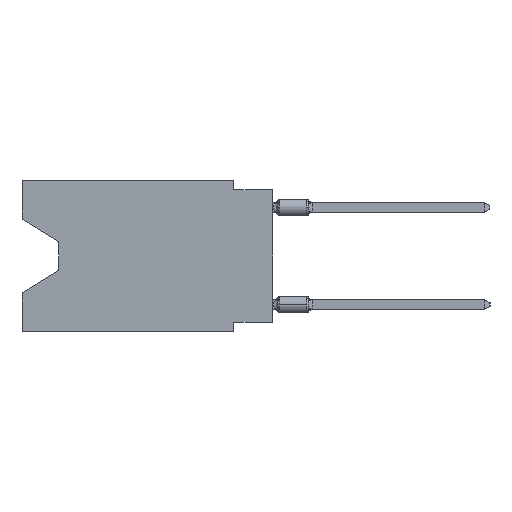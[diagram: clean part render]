
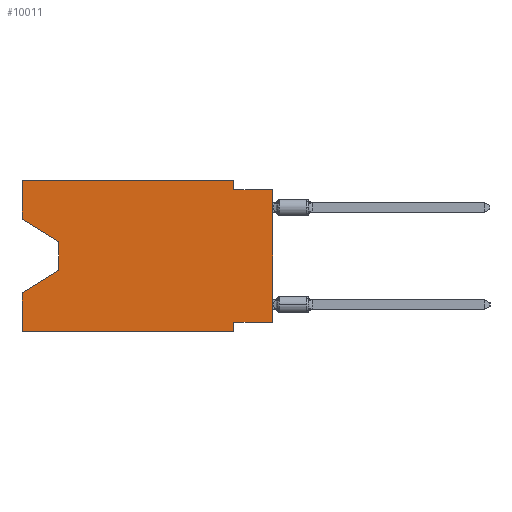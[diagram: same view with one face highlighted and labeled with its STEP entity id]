
A CAD part, left-side view. The second image highlights one B-rep face of the part: STEP entity #10011.
In plain terms, the highlighted planar face has unit normal (-1, 0, 0).
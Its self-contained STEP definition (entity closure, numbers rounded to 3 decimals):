
#190 = DIRECTION ( 'NONE',  ( 0., 0., 1. ) ) ;
#431 = DIRECTION ( 'NONE',  ( 0., -1., 0. ) ) ;
#808 = EDGE_CURVE ( 'NONE', #39180, #33706, #49292, .T. ) ;
#987 = CARTESIAN_POINT ( 'NONE',  ( 0., 16.383, -7.36 ) ) ;
#1009 = VERTEX_POINT ( 'NONE', #42931 ) ;
#2136 = ORIENTED_EDGE ( 'NONE', *, *, #48561, .F. ) ;
#2745 = VERTEX_POINT ( 'NONE', #40199 ) ;
#2796 = CARTESIAN_POINT ( 'NONE',  ( 0., 0., -9.271 ) ) ;
#2908 = LINE ( 'NONE', #24460, #17608 ) ;
#3637 = ORIENTED_EDGE ( 'NONE', *, *, #26050, .T. ) ;
#3849 = LINE ( 'NONE', #44059, #16710 ) ;
#6180 = ORIENTED_EDGE ( 'NONE', *, *, #808, .F. ) ;
#6496 = VECTOR ( 'NONE', #11713, 1000. ) ;
#6643 = VECTOR ( 'NONE', #20810, 1000. ) ;
#6736 = DIRECTION ( 'NONE',  ( 1., 0., 0. ) ) ;
#7237 = CARTESIAN_POINT ( 'NONE',  ( 0., 16.383, 0. ) ) ;
#7395 = DIRECTION ( 'NONE',  ( 0., -1., 0. ) ) ;
#8822 = EDGE_CURVE ( 'NONE', #22442, #29258, #32280, .T. ) ;
#8870 = CARTESIAN_POINT ( 'NONE',  ( 0., 16.383, 0. ) ) ;
#9523 = ORIENTED_EDGE ( 'NONE', *, *, #28208, .T. ) ;
#9620 = CARTESIAN_POINT ( 'NONE',  ( 0., 2.54, -0.635 ) ) ;
#10011 = ADVANCED_FACE ( 'NONE', ( #15449 ), #27844, .F. ) ;
#10468 = DIRECTION ( 'NONE',  ( 0., 0., 1. ) ) ;
#10819 = CARTESIAN_POINT ( 'NONE',  ( 0., 16.383, -9.906 ) ) ;
#11071 = VERTEX_POINT ( 'NONE', #987 ) ;
#11275 = EDGE_CURVE ( 'NONE', #22442, #39180, #39013, .T. ) ;
#11713 = DIRECTION ( 'NONE',  ( 0., -0.855, -0.519 ) ) ;
#11857 = CARTESIAN_POINT ( 'NONE',  ( 0., 16.383, 0. ) ) ;
#11991 = VECTOR ( 'NONE', #7395, 1000. ) ;
#11999 = CARTESIAN_POINT ( 'NONE',  ( 0., 2.54, -9.906 ) ) ;
#12377 = LINE ( 'NONE', #11857, #6643 ) ;
#12563 = ORIENTED_EDGE ( 'NONE', *, *, #39768, .F. ) ;
#12580 = ORIENTED_EDGE ( 'NONE', *, *, #33405, .F. ) ;
#13115 = DIRECTION ( 'NONE',  ( 0., 0.855, -0.519 ) ) ;
#14674 = ORIENTED_EDGE ( 'NONE', *, *, #8822, .T. ) ;
#14829 = CARTESIAN_POINT ( 'NONE',  ( 0., 16.383, -9.906 ) ) ;
#14930 = DIRECTION ( 'NONE',  ( 0., 0., -1. ) ) ;
#15289 = VECTOR ( 'NONE', #16594, 1000. ) ;
#15449 = FACE_OUTER_BOUND ( 'NONE', #28192, .T. ) ;
#15574 = VERTEX_POINT ( 'NONE', #10819 ) ;
#16594 = DIRECTION ( 'NONE',  ( 0., 0., -1. ) ) ;
#16710 = VECTOR ( 'NONE', #431, 1000. ) ;
#16806 = LINE ( 'NONE', #8870, #49374 ) ;
#17608 = VECTOR ( 'NONE', #13115, 1000. ) ;
#18321 = CARTESIAN_POINT ( 'NONE',  ( 0., 13.97, -5.893 ) ) ;
#18438 = CARTESIAN_POINT ( 'NONE',  ( 0., 0., -9.271 ) ) ;
#18748 = VERTEX_POINT ( 'NONE', #18321 ) ;
#19918 = DIRECTION ( 'NONE',  ( 0., 1., 0. ) ) ;
#20810 = DIRECTION ( 'NONE',  ( 0., -1., 0. ) ) ;
#21023 = EDGE_CURVE ( 'NONE', #29666, #2745, #16806, .T. ) ;
#21315 = CARTESIAN_POINT ( 'NONE',  ( 0., 16.383, -2.546 ) ) ;
#22442 = VERTEX_POINT ( 'NONE', #18438 ) ;
#24460 = CARTESIAN_POINT ( 'NONE',  ( 0., 13.97, -5.893 ) ) ;
#25561 = CARTESIAN_POINT ( 'NONE',  ( 0., 2.54, 0. ) ) ;
#26050 = EDGE_CURVE ( 'NONE', #18748, #11071, #2908, .T. ) ;
#27844 = PLANE ( 'NONE',  #36053 ) ;
#28137 = CARTESIAN_POINT ( 'NONE',  ( 0., 13.97, -4.013 ) ) ;
#28192 = EDGE_LOOP ( 'NONE', ( #40486, #9523, #3637, #2136, #48274, #6180, #35081, #14674, #12580, #12563, #45370, #38659 ) ) ;
#28208 = EDGE_CURVE ( 'NONE', #1009, #18748, #36070, .T. ) ;
#29258 = VERTEX_POINT ( 'NONE', #30095 ) ;
#29666 = VERTEX_POINT ( 'NONE', #21315 ) ;
#30095 = CARTESIAN_POINT ( 'NONE',  ( 0., 0., -0.635 ) ) ;
#30112 = EDGE_CURVE ( 'NONE', #15574, #33706, #47601, .T. ) ;
#30554 = LINE ( 'NONE', #46684, #32835 ) ;
#31979 = EDGE_CURVE ( 'NONE', #29666, #1009, #47662, .T. ) ;
#32280 = LINE ( 'NONE', #48403, #36812 ) ;
#32835 = VECTOR ( 'NONE', #10468, 1000. ) ;
#33405 = EDGE_CURVE ( 'NONE', #43121, #29258, #3849, .T. ) ;
#33706 = VERTEX_POINT ( 'NONE', #11999 ) ;
#33803 = VECTOR ( 'NONE', #33960, 1000. ) ;
#33960 = DIRECTION ( 'NONE',  ( 0., 0., -1. ) ) ;
#34191 = EDGE_CURVE ( 'NONE', #2745, #47792, #12377, .T. ) ;
#35081 = ORIENTED_EDGE ( 'NONE', *, *, #11275, .F. ) ;
#35461 = DIRECTION ( 'NONE',  ( 0., 0., 1. ) ) ;
#36053 = AXIS2_PLACEMENT_3D ( 'NONE', #7237, #6736, #14930 ) ;
#36070 = LINE ( 'NONE', #28137, #47307 ) ;
#36812 = VECTOR ( 'NONE', #35461, 1000. ) ;
#38659 = ORIENTED_EDGE ( 'NONE', *, *, #21023, .F. ) ;
#38753 = CARTESIAN_POINT ( 'NONE',  ( 0., 2.54, -9.271 ) ) ;
#38951 = CARTESIAN_POINT ( 'NONE',  ( 0., 2.54, 0. ) ) ;
#39013 = LINE ( 'NONE', #2796, #51337 ) ;
#39180 = VERTEX_POINT ( 'NONE', #38753 ) ;
#39768 = EDGE_CURVE ( 'NONE', #47792, #43121, #45159, .T. ) ;
#40064 = DIRECTION ( 'NONE',  ( 0., 0., -1. ) ) ;
#40199 = CARTESIAN_POINT ( 'NONE',  ( 0., 16.383, 0. ) ) ;
#40486 = ORIENTED_EDGE ( 'NONE', *, *, #31979, .T. ) ;
#42931 = CARTESIAN_POINT ( 'NONE',  ( 0., 13.97, -4.013 ) ) ;
#43121 = VERTEX_POINT ( 'NONE', #9620 ) ;
#44059 = CARTESIAN_POINT ( 'NONE',  ( 0., 0., -0.635 ) ) ;
#45159 = LINE ( 'NONE', #25561, #15289 ) ;
#45370 = ORIENTED_EDGE ( 'NONE', *, *, #34191, .F. ) ;
#46684 = CARTESIAN_POINT ( 'NONE',  ( 0., 16.383, 0. ) ) ;
#47307 = VECTOR ( 'NONE', #40064, 1000. ) ;
#47601 = LINE ( 'NONE', #14829, #11991 ) ;
#47662 = LINE ( 'NONE', #47915, #6496 ) ;
#47792 = VERTEX_POINT ( 'NONE', #38951 ) ;
#47915 = CARTESIAN_POINT ( 'NONE',  ( 0., 16.383, -2.546 ) ) ;
#48274 = ORIENTED_EDGE ( 'NONE', *, *, #30112, .T. ) ;
#48403 = CARTESIAN_POINT ( 'NONE',  ( 0., 0., 0. ) ) ;
#48561 = EDGE_CURVE ( 'NONE', #15574, #11071, #30554, .T. ) ;
#49292 = LINE ( 'NONE', #49808, #33803 ) ;
#49374 = VECTOR ( 'NONE', #190, 1000. ) ;
#49808 = CARTESIAN_POINT ( 'NONE',  ( 0., 2.54, -9.906 ) ) ;
#51337 = VECTOR ( 'NONE', #19918, 1000. ) ;
